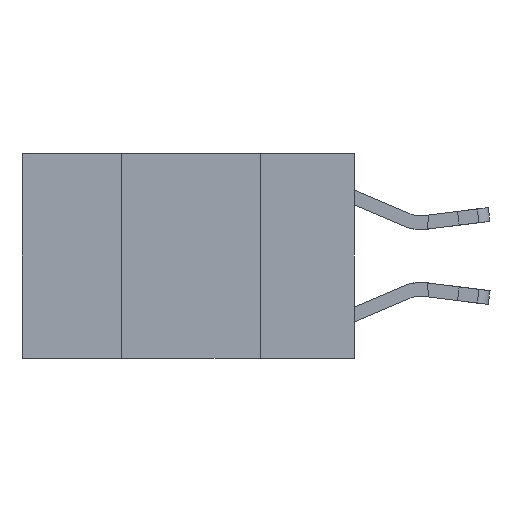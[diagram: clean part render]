
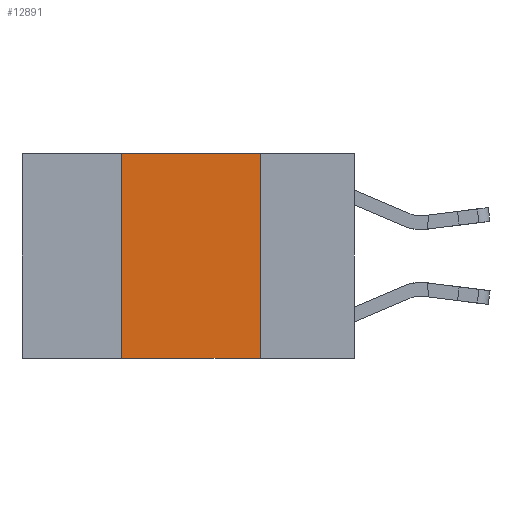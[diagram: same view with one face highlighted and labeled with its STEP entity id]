
A CAD part, left-side view. The second image highlights one B-rep face of the part: STEP entity #12891.
In plain terms, the highlighted planar face has unit normal (-1, 0, 0).
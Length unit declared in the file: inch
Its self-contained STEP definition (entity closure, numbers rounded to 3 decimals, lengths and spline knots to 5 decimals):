
#292 = EDGE_LOOP ( 'NONE', ( #8163, #4516, #15755, #6081 ) ) ;
#333 = VECTOR ( 'NONE', #11766, 39.37008 ) ;
#748 = LINE ( 'NONE', #6535, #333 ) ;
#1503 = DIRECTION ( 'NONE',  ( 0., -1., 0. ) ) ;
#1580 = DIRECTION ( 'NONE',  ( 1., 0., 0. ) ) ;
#2133 = EDGE_CURVE ( 'NONE', #12311, #5455, #7592, .T. ) ;
#2236 = DIRECTION ( 'NONE',  ( 0., 0., 1. ) ) ;
#3232 = AXIS2_PLACEMENT_3D ( 'NONE', #9447, #1580, #10765 ) ;
#3956 = EDGE_CURVE ( 'NONE', #10767, #12311, #13759, .T. ) ;
#4516 = ORIENTED_EDGE ( 'NONE', *, *, #2133, .F. ) ;
#4600 = EDGE_CURVE ( 'NONE', #5455, #4785, #748, .T. ) ;
#4785 = VERTEX_POINT ( 'NONE', #9523 ) ;
#4798 = FACE_OUTER_BOUND ( 'NONE', #292, .T. ) ;
#5259 = EDGE_CURVE ( 'NONE', #10767, #4785, #15345, .T. ) ;
#5455 = VERTEX_POINT ( 'NONE', #14041 ) ;
#6081 = ORIENTED_EDGE ( 'NONE', *, *, #5259, .T. ) ;
#6535 = CARTESIAN_POINT ( 'NONE',  ( 0., 0.17, 0. ) ) ;
#6722 = CARTESIAN_POINT ( 'NONE',  ( 0., 0.6, 0. ) ) ;
#6742 = VECTOR ( 'NONE', #2236, 39.37008 ) ;
#7592 = LINE ( 'NONE', #6722, #14227 ) ;
#8163 = ORIENTED_EDGE ( 'NONE', *, *, #4600, .F. ) ;
#8317 = VECTOR ( 'NONE', #12130, 39.37008 ) ;
#8838 = CARTESIAN_POINT ( 'NONE',  ( 0., 0.42, 0. ) ) ;
#9447 = CARTESIAN_POINT ( 'NONE',  ( 0., 0.6, 0. ) ) ;
#9523 = CARTESIAN_POINT ( 'NONE',  ( 0., 0.17, -0.37 ) ) ;
#10765 = DIRECTION ( 'NONE',  ( 0., 0., -1. ) ) ;
#10767 = VERTEX_POINT ( 'NONE', #13541 ) ;
#10790 = CARTESIAN_POINT ( 'NONE',  ( 0., 0.6, -0.37 ) ) ;
#10840 = CARTESIAN_POINT ( 'NONE',  ( 0., 0.42, 0. ) ) ;
#11766 = DIRECTION ( 'NONE',  ( 0., 0., -1. ) ) ;
#12130 = DIRECTION ( 'NONE',  ( 0., -1., 0. ) ) ;
#12311 = VERTEX_POINT ( 'NONE', #10840 ) ;
#12891 = ADVANCED_FACE ( 'NONE', ( #4798 ), #16002, .F. ) ;
#13541 = CARTESIAN_POINT ( 'NONE',  ( 0., 0.42, -0.37 ) ) ;
#13759 = LINE ( 'NONE', #8838, #6742 ) ;
#14041 = CARTESIAN_POINT ( 'NONE',  ( 0., 0.17, 0. ) ) ;
#14227 = VECTOR ( 'NONE', #1503, 39.37008 ) ;
#15345 = LINE ( 'NONE', #10790, #8317 ) ;
#15755 = ORIENTED_EDGE ( 'NONE', *, *, #3956, .F. ) ;
#16002 = PLANE ( 'NONE',  #3232 ) ;
